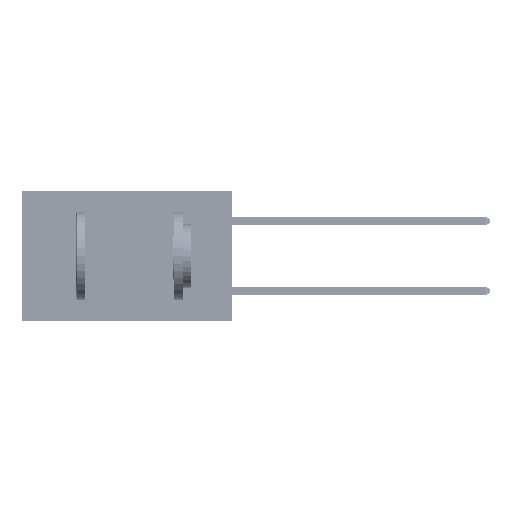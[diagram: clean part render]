
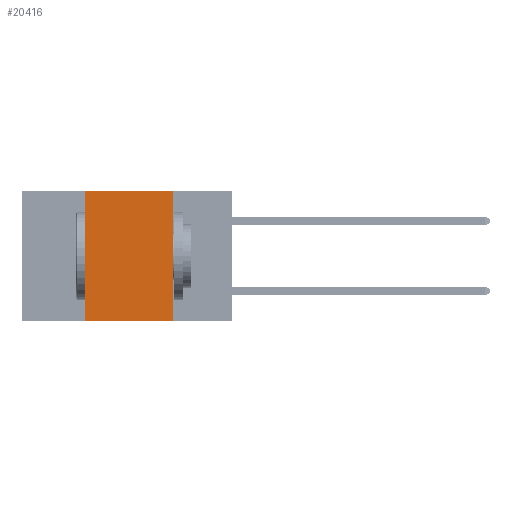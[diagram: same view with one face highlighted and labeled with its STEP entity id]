
A CAD part, left-side view. The second image highlights one B-rep face of the part: STEP entity #20416.
In plain terms, the highlighted planar face has unit normal (-1, 0, 0).
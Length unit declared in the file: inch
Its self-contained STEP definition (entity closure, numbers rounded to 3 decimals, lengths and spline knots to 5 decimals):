
#766 = CARTESIAN_POINT ( 'NONE',  ( 0., 0.6, 0. ) ) ;
#1094 = DIRECTION ( 'NONE',  ( 1., 0., 0. ) ) ;
#1256 = CARTESIAN_POINT ( 'NONE',  ( 0., 0.6, 0. ) ) ;
#2019 = ORIENTED_EDGE ( 'NONE', *, *, #46185, .T. ) ;
#2529 = LINE ( 'NONE', #766, #45967 ) ;
#3334 = DIRECTION ( 'NONE',  ( 0., 0., -1. ) ) ;
#3415 = VERTEX_POINT ( 'NONE', #27858 ) ;
#5474 = CARTESIAN_POINT ( 'NONE',  ( 0., 0.42, 0. ) ) ;
#7733 = LINE ( 'NONE', #42557, #14123 ) ;
#8027 = ORIENTED_EDGE ( 'NONE', *, *, #14580, .F. ) ;
#10196 = EDGE_CURVE ( 'NONE', #40848, #33990, #18945, .T. ) ;
#14123 = VECTOR ( 'NONE', #27483, 39.37008 ) ;
#14580 = EDGE_CURVE ( 'NONE', #36878, #40848, #2529, .T. ) ;
#14583 = CARTESIAN_POINT ( 'NONE',  ( 0., 0.17, -0.37 ) ) ;
#18366 = LINE ( 'NONE', #38668, #41611 ) ;
#18945 = LINE ( 'NONE', #47818, #35803 ) ;
#20416 = ADVANCED_FACE ( 'NONE', ( #21266 ), #31241, .F. ) ;
#21266 = FACE_OUTER_BOUND ( 'NONE', #24220, .T. ) ;
#24220 = EDGE_LOOP ( 'NONE', ( #43064, #8027, #44734, #2019 ) ) ;
#24334 = AXIS2_PLACEMENT_3D ( 'NONE', #1256, #1094, #42284 ) ;
#25066 = EDGE_CURVE ( 'NONE', #3415, #36878, #18366, .T. ) ;
#27483 = DIRECTION ( 'NONE',  ( 0., -1., 0. ) ) ;
#27651 = CARTESIAN_POINT ( 'NONE',  ( 0., 0.17, 0. ) ) ;
#27858 = CARTESIAN_POINT ( 'NONE',  ( 0., 0.42, -0.37 ) ) ;
#31241 = PLANE ( 'NONE',  #24334 ) ;
#33990 = VERTEX_POINT ( 'NONE', #14583 ) ;
#35132 = DIRECTION ( 'NONE',  ( 0., -1., 0. ) ) ;
#35250 = DIRECTION ( 'NONE',  ( 0., 0., 1. ) ) ;
#35803 = VECTOR ( 'NONE', #3334, 39.37008 ) ;
#36878 = VERTEX_POINT ( 'NONE', #5474 ) ;
#38668 = CARTESIAN_POINT ( 'NONE',  ( 0., 0.42, 0. ) ) ;
#40848 = VERTEX_POINT ( 'NONE', #27651 ) ;
#41611 = VECTOR ( 'NONE', #35250, 39.37008 ) ;
#42284 = DIRECTION ( 'NONE',  ( 0., 0., -1. ) ) ;
#42557 = CARTESIAN_POINT ( 'NONE',  ( 0., 0.6, -0.37 ) ) ;
#43064 = ORIENTED_EDGE ( 'NONE', *, *, #10196, .F. ) ;
#44734 = ORIENTED_EDGE ( 'NONE', *, *, #25066, .F. ) ;
#45967 = VECTOR ( 'NONE', #35132, 39.37008 ) ;
#46185 = EDGE_CURVE ( 'NONE', #3415, #33990, #7733, .T. ) ;
#47818 = CARTESIAN_POINT ( 'NONE',  ( 0., 0.17, 0. ) ) ;
